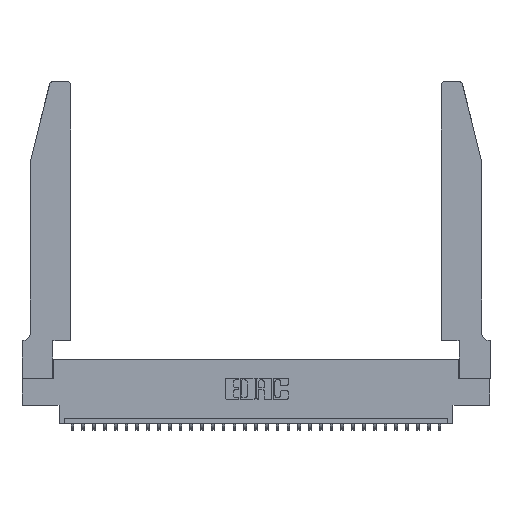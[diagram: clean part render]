
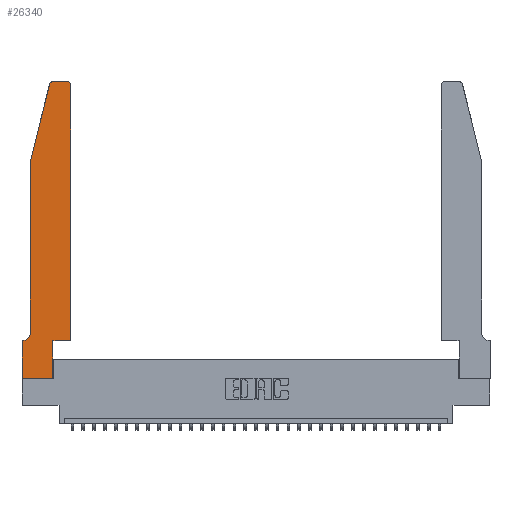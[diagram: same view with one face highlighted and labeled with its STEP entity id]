
A CAD part, top view. The second image highlights one B-rep face of the part: STEP entity #26340.
In plain terms, the highlighted planar face has unit normal (0, 0, 1).
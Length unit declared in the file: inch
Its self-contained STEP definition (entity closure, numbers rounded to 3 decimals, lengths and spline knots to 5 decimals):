
#179 = CARTESIAN_POINT ( 'NONE',  ( 0.2605, 2.75, 0.37 ) ) ;
#279 = DIRECTION ( 'NONE',  ( 0., 1., 0. ) ) ;
#290 = FACE_OUTER_BOUND ( 'NONE', #18419, .T. ) ;
#371 = VERTEX_POINT ( 'NONE', #14500 ) ;
#724 = CARTESIAN_POINT ( 'NONE',  ( 0.4505, 0.35, 0.37 ) ) ;
#902 = CARTESIAN_POINT ( 'NONE',  ( 0., 0., 0.37 ) ) ;
#1480 = VECTOR ( 'NONE', #279, 39.37008 ) ;
#1484 = CARTESIAN_POINT ( 'NONE',  ( 0., 0.35, 0.37 ) ) ;
#2173 = VERTEX_POINT ( 'NONE', #29748 ) ;
#2570 = CARTESIAN_POINT ( 'NONE',  ( 0.0755, 2., 0.37 ) ) ;
#2695 = EDGE_CURVE ( 'NONE', #6441, #6920, #20012, .T. ) ;
#3143 = CARTESIAN_POINT ( 'NONE',  ( 0.2865, 0.35, 0.37 ) ) ;
#3166 = CARTESIAN_POINT ( 'NONE',  ( 0.0755, 2., 0.37 ) ) ;
#3572 = DIRECTION ( 'NONE',  ( 0., 0., 1. ) ) ;
#3615 = CARTESIAN_POINT ( 'NONE',  ( 0., 0., 0.37 ) ) ;
#3943 = LINE ( 'NONE', #10571, #31219 ) ;
#4454 = CARTESIAN_POINT ( 'NONE',  ( 0.0755, 0.42, 0.37 ) ) ;
#4860 = CARTESIAN_POINT ( 'NONE',  ( 0., 0., 0.37 ) ) ;
#5448 = EDGE_CURVE ( 'NONE', #12167, #12798, #30591, .T. ) ;
#6108 = ORIENTED_EDGE ( 'NONE', *, *, #26708, .T. ) ;
#6233 = DIRECTION ( 'NONE',  ( 0., -1., 0. ) ) ;
#6441 = VERTEX_POINT ( 'NONE', #14260 ) ;
#6920 = VERTEX_POINT ( 'NONE', #3166 ) ;
#6922 = LINE ( 'NONE', #179, #20568 ) ;
#7071 = AXIS2_PLACEMENT_3D ( 'NONE', #31127, #3572, #26260 ) ;
#7375 = CARTESIAN_POINT ( 'NONE',  ( 0.0755, 2., 0.37 ) ) ;
#8089 = LINE ( 'NONE', #28874, #1480 ) ;
#8384 = DIRECTION ( 'NONE',  ( 1., 0., 0. ) ) ;
#8655 = CIRCLE ( 'NONE', #7071, 0.03 ) ;
#8734 = EDGE_CURVE ( 'NONE', #27810, #12025, #3943, .T. ) ;
#10056 = EDGE_CURVE ( 'NONE', #2173, #6441, #10474, .T. ) ;
#10474 = CIRCLE ( 'NONE', #27854, 0.03 ) ;
#10571 = CARTESIAN_POINT ( 'NONE',  ( 0.4505, 0.35, 0.37 ) ) ;
#10625 = LINE ( 'NONE', #7375, #27365 ) ;
#10760 = VECTOR ( 'NONE', #6233, 39.37008 ) ;
#11010 = CARTESIAN_POINT ( 'NONE',  ( 0.2865, 0.35, 0.37 ) ) ;
#11559 = VECTOR ( 'NONE', #18912, 39.37008 ) ;
#11571 = EDGE_CURVE ( 'NONE', #20201, #24697, #28252, .T. ) ;
#11716 = ORIENTED_EDGE ( 'NONE', *, *, #18732, .T. ) ;
#11768 = EDGE_CURVE ( 'NONE', #24697, #12167, #25956, .T. ) ;
#12025 = VERTEX_POINT ( 'NONE', #724 ) ;
#12114 = DIRECTION ( 'NONE',  ( 1., 0., 0. ) ) ;
#12167 = VERTEX_POINT ( 'NONE', #3615 ) ;
#12798 = VERTEX_POINT ( 'NONE', #30942 ) ;
#12944 = VERTEX_POINT ( 'NONE', #31974 ) ;
#13154 = PLANE ( 'NONE',  #19845 ) ;
#13278 = EDGE_CURVE ( 'NONE', #6920, #29583, #10625, .T. ) ;
#13578 = EDGE_CURVE ( 'NONE', #371, #12944, #8655, .T. ) ;
#14169 = CARTESIAN_POINT ( 'NONE',  ( 0.0055, 0.35, 0.37 ) ) ;
#14260 = CARTESIAN_POINT ( 'NONE',  ( 0.25487, 2.72718, 0.37 ) ) ;
#14500 = CARTESIAN_POINT ( 'NONE',  ( 0.4505, 2.72, 0.37 ) ) ;
#14603 = DIRECTION ( 'NONE',  ( 0., 0., 1. ) ) ;
#14924 = DIRECTION ( 'NONE',  ( -0.239, -0.971, 0. ) ) ;
#16984 = CARTESIAN_POINT ( 'NONE',  ( 0.284, 2.72, 0.37 ) ) ;
#17084 = ORIENTED_EDGE ( 'NONE', *, *, #11768, .T. ) ;
#17104 = DIRECTION ( 'NONE',  ( 0., -1., 0. ) ) ;
#17726 = DIRECTION ( 'NONE',  ( -1., 0., 0. ) ) ;
#18419 = EDGE_LOOP ( 'NONE', ( #22537, #18455, #23491, #32234, #11716, #21115, #17084, #26543, #21941, #28278, #6108, #29329 ) ) ;
#18455 = ORIENTED_EDGE ( 'NONE', *, *, #10056, .T. ) ;
#18732 = EDGE_CURVE ( 'NONE', #29583, #20201, #30544, .T. ) ;
#18866 = CARTESIAN_POINT ( 'NONE',  ( 0.0055, 0.42, 0.37 ) ) ;
#18912 = DIRECTION ( 'NONE',  ( -1., 0., 0. ) ) ;
#19187 = DIRECTION ( 'NONE',  ( -1., 0., 0. ) ) ;
#19845 = AXIS2_PLACEMENT_3D ( 'NONE', #30505, #23377, #31293 ) ;
#20012 = LINE ( 'NONE', #2570, #29718 ) ;
#20201 = VERTEX_POINT ( 'NONE', #14169 ) ;
#20568 = VECTOR ( 'NONE', #17726, 39.37008 ) ;
#20957 = VECTOR ( 'NONE', #28168, 39.37008 ) ;
#21115 = ORIENTED_EDGE ( 'NONE', *, *, #11571, .T. ) ;
#21941 = ORIENTED_EDGE ( 'NONE', *, *, #23171, .T. ) ;
#22302 = DIRECTION ( 'NONE',  ( 1., 0., 0. ) ) ;
#22537 = ORIENTED_EDGE ( 'NONE', *, *, #26634, .T. ) ;
#23171 = EDGE_CURVE ( 'NONE', #12798, #27810, #31050, .T. ) ;
#23377 = DIRECTION ( 'NONE',  ( 0., 0., 1. ) ) ;
#23491 = ORIENTED_EDGE ( 'NONE', *, *, #2695, .T. ) ;
#24019 = VECTOR ( 'NONE', #22302, 39.37008 ) ;
#24697 = VERTEX_POINT ( 'NONE', #1484 ) ;
#25956 = LINE ( 'NONE', #902, #10760 ) ;
#26260 = DIRECTION ( 'NONE',  ( 1., 0., 0. ) ) ;
#26340 = ADVANCED_FACE ( 'NONE', ( #290 ), #13154, .T. ) ;
#26543 = ORIENTED_EDGE ( 'NONE', *, *, #5448, .T. ) ;
#26634 = EDGE_CURVE ( 'NONE', #12944, #2173, #6922, .T. ) ;
#26708 = EDGE_CURVE ( 'NONE', #12025, #371, #8089, .T. ) ;
#26984 = AXIS2_PLACEMENT_3D ( 'NONE', #18866, #31549, #19187 ) ;
#27365 = VECTOR ( 'NONE', #17104, 39.37008 ) ;
#27810 = VERTEX_POINT ( 'NONE', #3143 ) ;
#27854 = AXIS2_PLACEMENT_3D ( 'NONE', #16984, #14603, #12114 ) ;
#27901 = CARTESIAN_POINT ( 'NONE',  ( 0.0755, 0.35, 0.37 ) ) ;
#28168 = DIRECTION ( 'NONE',  ( 0., 1., 0. ) ) ;
#28252 = LINE ( 'NONE', #27901, #11559 ) ;
#28278 = ORIENTED_EDGE ( 'NONE', *, *, #8734, .T. ) ;
#28874 = CARTESIAN_POINT ( 'NONE',  ( 0.4505, 0.35, 0.37 ) ) ;
#29329 = ORIENTED_EDGE ( 'NONE', *, *, #13578, .T. ) ;
#29583 = VERTEX_POINT ( 'NONE', #4454 ) ;
#29718 = VECTOR ( 'NONE', #14924, 39.37008 ) ;
#29748 = CARTESIAN_POINT ( 'NONE',  ( 0.284, 2.75, 0.37 ) ) ;
#30505 = CARTESIAN_POINT ( 'NONE',  ( 0., 0.35, 0.37 ) ) ;
#30544 = CIRCLE ( 'NONE', #26984, 0.07 ) ;
#30591 = LINE ( 'NONE', #4860, #24019 ) ;
#30942 = CARTESIAN_POINT ( 'NONE',  ( 0.2865, 0., 0.37 ) ) ;
#31050 = LINE ( 'NONE', #11010, #20957 ) ;
#31127 = CARTESIAN_POINT ( 'NONE',  ( 0.4205, 2.72, 0.37 ) ) ;
#31219 = VECTOR ( 'NONE', #8384, 39.37008 ) ;
#31293 = DIRECTION ( 'NONE',  ( 1., 0., 0. ) ) ;
#31549 = DIRECTION ( 'NONE',  ( 0., 0., -1. ) ) ;
#31974 = CARTESIAN_POINT ( 'NONE',  ( 0.4205, 2.75, 0.37 ) ) ;
#32234 = ORIENTED_EDGE ( 'NONE', *, *, #13278, .T. ) ;
